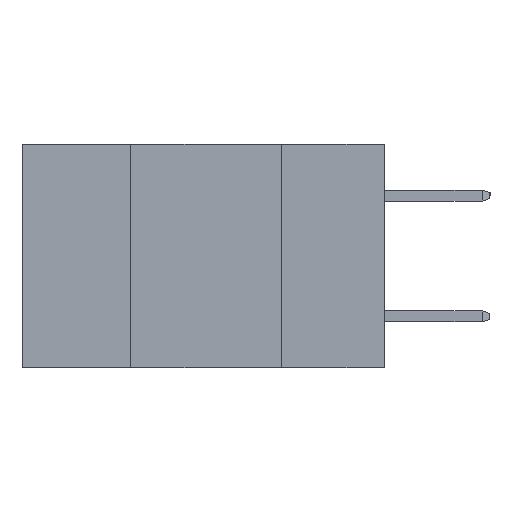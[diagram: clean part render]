
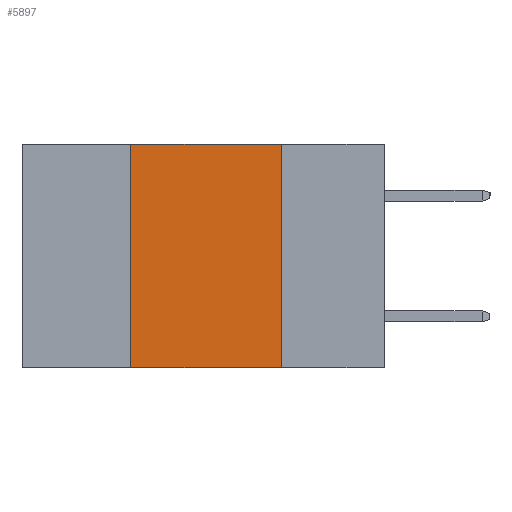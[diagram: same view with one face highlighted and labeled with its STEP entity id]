
A CAD part, left-side view. The second image highlights one B-rep face of the part: STEP entity #5897.
In plain terms, the highlighted planar face has unit normal (-1, 0, 0).
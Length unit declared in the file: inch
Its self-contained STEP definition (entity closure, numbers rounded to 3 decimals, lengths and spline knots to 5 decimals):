
#281 = LINE ( 'NONE', #16946, #5850 ) ;
#451 = CARTESIAN_POINT ( 'NONE',  ( 0., 0.42, -0.37 ) ) ;
#1130 = CARTESIAN_POINT ( 'NONE',  ( 0., 0.6, 0. ) ) ;
#1630 = VERTEX_POINT ( 'NONE', #18766 ) ;
#2012 = CARTESIAN_POINT ( 'NONE',  ( 0., 0.17, 0. ) ) ;
#2739 = CARTESIAN_POINT ( 'NONE',  ( 0., 0.6, 0. ) ) ;
#2777 = EDGE_CURVE ( 'NONE', #19614, #4506, #281, .T. ) ;
#2874 = DIRECTION ( 'NONE',  ( 0., -1., 0. ) ) ;
#2978 = AXIS2_PLACEMENT_3D ( 'NONE', #2739, #13604, #11571 ) ;
#4227 = CARTESIAN_POINT ( 'NONE',  ( 0., 0.6, -0.37 ) ) ;
#4295 = PLANE ( 'NONE',  #2978 ) ;
#4320 = ORIENTED_EDGE ( 'NONE', *, *, #9006, .F. ) ;
#4359 = CARTESIAN_POINT ( 'NONE',  ( 0., 0.17, -0.37 ) ) ;
#4506 = VERTEX_POINT ( 'NONE', #4359 ) ;
#4765 = ORIENTED_EDGE ( 'NONE', *, *, #2777, .F. ) ;
#5850 = VECTOR ( 'NONE', #7693, 39.37008 ) ;
#5897 = ADVANCED_FACE ( 'NONE', ( #11777 ), #4295, .F. ) ;
#6002 = VECTOR ( 'NONE', #16591, 39.37008 ) ;
#6523 = CARTESIAN_POINT ( 'NONE',  ( 0., 0.42, 0. ) ) ;
#6539 = DIRECTION ( 'NONE',  ( 0., 0., 1. ) ) ;
#7693 = DIRECTION ( 'NONE',  ( 0., 0., -1. ) ) ;
#8122 = ORIENTED_EDGE ( 'NONE', *, *, #18666, .T. ) ;
#8839 = VERTEX_POINT ( 'NONE', #6523 ) ;
#9006 = EDGE_CURVE ( 'NONE', #8839, #19614, #13524, .T. ) ;
#11571 = DIRECTION ( 'NONE',  ( 0., 0., -1. ) ) ;
#11777 = FACE_OUTER_BOUND ( 'NONE', #14810, .T. ) ;
#13524 = LINE ( 'NONE', #1130, #15682 ) ;
#13604 = DIRECTION ( 'NONE',  ( 1., 0., 0. ) ) ;
#14624 = EDGE_CURVE ( 'NONE', #1630, #8839, #17609, .T. ) ;
#14810 = EDGE_LOOP ( 'NONE', ( #4765, #4320, #14813, #8122 ) ) ;
#14813 = ORIENTED_EDGE ( 'NONE', *, *, #14624, .F. ) ;
#15682 = VECTOR ( 'NONE', #2874, 39.37008 ) ;
#15840 = VECTOR ( 'NONE', #6539, 39.37008 ) ;
#16591 = DIRECTION ( 'NONE',  ( 0., -1., 0. ) ) ;
#16946 = CARTESIAN_POINT ( 'NONE',  ( 0., 0.17, -0.37 ) ) ;
#17609 = LINE ( 'NONE', #451, #15840 ) ;
#18120 = LINE ( 'NONE', #4227, #6002 ) ;
#18666 = EDGE_CURVE ( 'NONE', #1630, #4506, #18120, .T. ) ;
#18766 = CARTESIAN_POINT ( 'NONE',  ( 0., 0.42, -0.37 ) ) ;
#19614 = VERTEX_POINT ( 'NONE', #2012 ) ;
